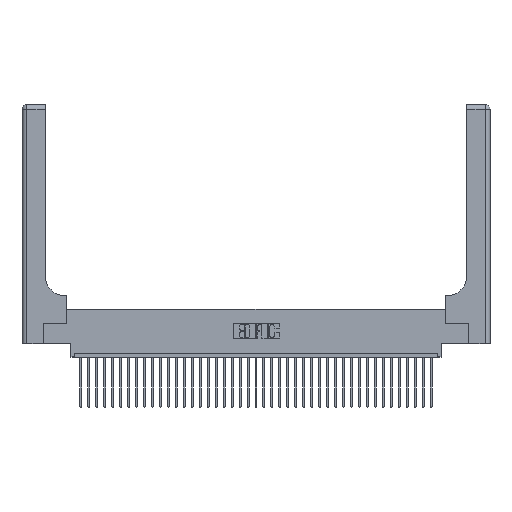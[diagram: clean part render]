
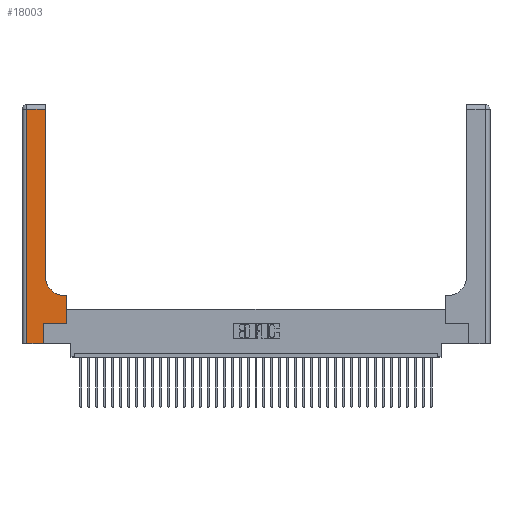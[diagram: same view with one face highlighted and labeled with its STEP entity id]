
A CAD part, top view. The second image highlights one B-rep face of the part: STEP entity #18003.
In plain terms, the highlighted planar face has unit normal (0, 0, 1).
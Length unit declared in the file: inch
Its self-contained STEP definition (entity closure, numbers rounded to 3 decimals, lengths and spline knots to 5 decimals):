
#137 = ORIENTED_EDGE ( 'NONE', *, *, #31783, .T. ) ;
#138 = VERTEX_POINT ( 'NONE', #7788 ) ;
#461 = EDGE_CURVE ( 'NONE', #12718, #21491, #37431, .T. ) ;
#570 = ORIENTED_EDGE ( 'NONE', *, *, #461, .T. ) ;
#586 = VECTOR ( 'NONE', #32729, 39.37008 ) ;
#673 = EDGE_CURVE ( 'NONE', #34341, #10572, #32326, .T. ) ;
#738 = LINE ( 'NONE', #4683, #38272 ) ;
#916 = ORIENTED_EDGE ( 'NONE', *, *, #7121, .T. ) ;
#973 = ORIENTED_EDGE ( 'NONE', *, *, #14071, .T. ) ;
#1164 = CARTESIAN_POINT ( 'NONE',  ( 0., 0., 0.37 ) ) ;
#1821 = CARTESIAN_POINT ( 'NONE',  ( 0.2915, 2.94, 0.37 ) ) ;
#2536 = LINE ( 'NONE', #32855, #586 ) ;
#3576 = DIRECTION ( 'NONE',  ( 0., 1., 0. ) ) ;
#4683 = CARTESIAN_POINT ( 'NONE',  ( 0.2915, 3., 0.37 ) ) ;
#6799 = CARTESIAN_POINT ( 'NONE',  ( 0.5585, 0.25, 0.37 ) ) ;
#6923 = ORIENTED_EDGE ( 'NONE', *, *, #673, .T. ) ;
#7121 = EDGE_CURVE ( 'NONE', #138, #12718, #8986, .T. ) ;
#7218 = AXIS2_PLACEMENT_3D ( 'NONE', #34092, #13137, #16895 ) ;
#7246 = LINE ( 'NONE', #12150, #7773 ) ;
#7547 = VECTOR ( 'NONE', #37267, 39.37008 ) ;
#7773 = VECTOR ( 'NONE', #36223, 39.37008 ) ;
#7788 = CARTESIAN_POINT ( 'NONE',  ( 0.06, 2.94, 0.37 ) ) ;
#7993 = DIRECTION ( 'NONE',  ( 0., 1., 0. ) ) ;
#8986 = LINE ( 'NONE', #28247, #7547 ) ;
#9148 = DIRECTION ( 'NONE',  ( 1., 0., 0. ) ) ;
#9382 = ORIENTED_EDGE ( 'NONE', *, *, #33242, .T. ) ;
#10572 = VERTEX_POINT ( 'NONE', #38148 ) ;
#10672 = CARTESIAN_POINT ( 'NONE',  ( 0.5415, 0.6, 0.37 ) ) ;
#10955 = VERTEX_POINT ( 'NONE', #1821 ) ;
#12150 = CARTESIAN_POINT ( 'NONE',  ( 0., 2.94, 0.37 ) ) ;
#12532 = LINE ( 'NONE', #30963, #14486 ) ;
#12718 = VERTEX_POINT ( 'NONE', #33743 ) ;
#13137 = DIRECTION ( 'NONE',  ( 0., 0., -1. ) ) ;
#13475 = CARTESIAN_POINT ( 'NONE',  ( 0.269, 0.25, 0.37 ) ) ;
#14071 = EDGE_CURVE ( 'NONE', #21491, #24854, #16066, .T. ) ;
#14448 = CARTESIAN_POINT ( 'NONE',  ( 0.5585, 0.6, 0.37 ) ) ;
#14486 = VECTOR ( 'NONE', #3576, 39.37008 ) ;
#16066 = LINE ( 'NONE', #28194, #28757 ) ;
#16241 = CARTESIAN_POINT ( 'NONE',  ( 0.269, 0., 0.37 ) ) ;
#16895 = DIRECTION ( 'NONE',  ( 1., 0., 0. ) ) ;
#18003 = ADVANCED_FACE ( 'NONE', ( #20025 ), #38307, .F. ) ;
#20025 = FACE_OUTER_BOUND ( 'NONE', #33470, .T. ) ;
#21461 = VECTOR ( 'NONE', #31291, 39.37008 ) ;
#21491 = VERTEX_POINT ( 'NONE', #16241 ) ;
#22364 = EDGE_CURVE ( 'NONE', #24854, #24816, #34003, .T. ) ;
#22632 = AXIS2_PLACEMENT_3D ( 'NONE', #29761, #35404, #38432 ) ;
#24025 = ORIENTED_EDGE ( 'NONE', *, *, #25653, .T. ) ;
#24196 = VECTOR ( 'NONE', #9148, 39.37008 ) ;
#24816 = VERTEX_POINT ( 'NONE', #6799 ) ;
#24854 = VERTEX_POINT ( 'NONE', #13475 ) ;
#25653 = EDGE_CURVE ( 'NONE', #10955, #138, #7246, .T. ) ;
#25764 = DIRECTION ( 'NONE',  ( 0., 1., 0. ) ) ;
#27642 = ORIENTED_EDGE ( 'NONE', *, *, #22364, .T. ) ;
#28194 = CARTESIAN_POINT ( 'NONE',  ( 0.269, 0., 0.37 ) ) ;
#28247 = CARTESIAN_POINT ( 'NONE',  ( 0.06, 3., 0.37 ) ) ;
#28757 = VECTOR ( 'NONE', #25764, 39.37008 ) ;
#29761 = CARTESIAN_POINT ( 'NONE',  ( 0., 3., 0.37 ) ) ;
#30963 = CARTESIAN_POINT ( 'NONE',  ( 0.5585, 0.25, 0.37 ) ) ;
#31291 = DIRECTION ( 'NONE',  ( 1., 0., 0. ) ) ;
#31783 = EDGE_CURVE ( 'NONE', #10572, #10955, #738, .T. ) ;
#32251 = CARTESIAN_POINT ( 'NONE',  ( 0.269, 0.25, 0.37 ) ) ;
#32326 = CIRCLE ( 'NONE', #7218, 0.25 ) ;
#32528 = VERTEX_POINT ( 'NONE', #14448 ) ;
#32729 = DIRECTION ( 'NONE',  ( -1., 0., 0. ) ) ;
#32855 = CARTESIAN_POINT ( 'NONE',  ( 0.2915, 0.6, 0.37 ) ) ;
#33242 = EDGE_CURVE ( 'NONE', #32528, #34341, #2536, .T. ) ;
#33470 = EDGE_LOOP ( 'NONE', ( #137, #24025, #916, #570, #973, #27642, #34176, #9382, #6923 ) ) ;
#33743 = CARTESIAN_POINT ( 'NONE',  ( 0.06, 0., 0.37 ) ) ;
#34003 = LINE ( 'NONE', #32251, #24196 ) ;
#34092 = CARTESIAN_POINT ( 'NONE',  ( 0.5415, 0.85, 0.37 ) ) ;
#34176 = ORIENTED_EDGE ( 'NONE', *, *, #36355, .T. ) ;
#34341 = VERTEX_POINT ( 'NONE', #10672 ) ;
#35404 = DIRECTION ( 'NONE',  ( 0., 0., -1. ) ) ;
#36223 = DIRECTION ( 'NONE',  ( -1., 0., 0. ) ) ;
#36355 = EDGE_CURVE ( 'NONE', #24816, #32528, #12532, .T. ) ;
#37267 = DIRECTION ( 'NONE',  ( 0., -1., 0. ) ) ;
#37431 = LINE ( 'NONE', #1164, #21461 ) ;
#38148 = CARTESIAN_POINT ( 'NONE',  ( 0.2915, 0.85, 0.37 ) ) ;
#38272 = VECTOR ( 'NONE', #7993, 39.37008 ) ;
#38307 = PLANE ( 'NONE',  #22632 ) ;
#38432 = DIRECTION ( 'NONE',  ( -1., 0., 0. ) ) ;
